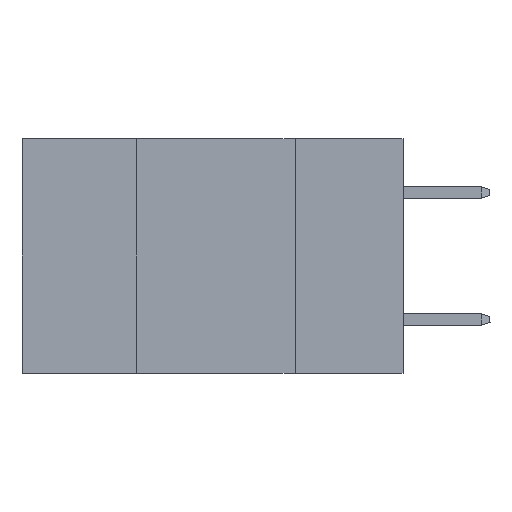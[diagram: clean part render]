
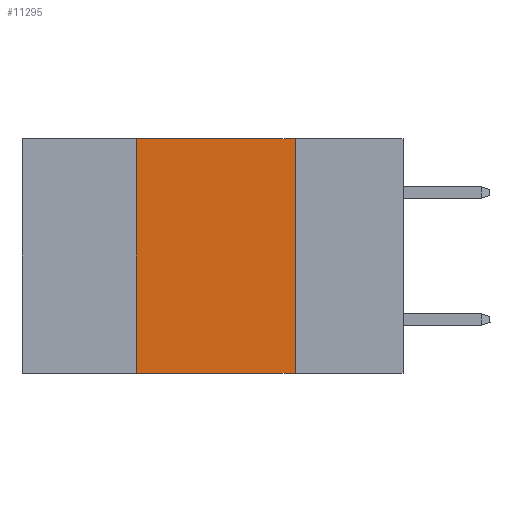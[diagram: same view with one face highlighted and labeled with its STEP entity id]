
A CAD part, left-side view. The second image highlights one B-rep face of the part: STEP entity #11295.
In plain terms, the highlighted planar face has unit normal (-1, 0, 0).
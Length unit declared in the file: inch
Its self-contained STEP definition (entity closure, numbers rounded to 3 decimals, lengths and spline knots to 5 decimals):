
#46 = CARTESIAN_POINT ( 'NONE',  ( 0., 0.42, -0.37 ) ) ;
#271 = ORIENTED_EDGE ( 'NONE', *, *, #1287, .F. ) ;
#534 = CARTESIAN_POINT ( 'NONE',  ( 0., 0.17, -0.37 ) ) ;
#814 = LINE ( 'NONE', #4712, #7866 ) ;
#1287 = EDGE_CURVE ( 'NONE', #6392, #10221, #2279, .T. ) ;
#1678 = CARTESIAN_POINT ( 'NONE',  ( 0., 0.6, 0. ) ) ;
#2162 = EDGE_LOOP ( 'NONE', ( #271, #5222, #3661, #5683 ) ) ;
#2279 = LINE ( 'NONE', #11916, #7397 ) ;
#2677 = LINE ( 'NONE', #10434, #7448 ) ;
#3661 = ORIENTED_EDGE ( 'NONE', *, *, #4582, .F. ) ;
#3765 = CARTESIAN_POINT ( 'NONE',  ( 0., 0.17, 0. ) ) ;
#4069 = VERTEX_POINT ( 'NONE', #46 ) ;
#4582 = EDGE_CURVE ( 'NONE', #4069, #7107, #12028, .T. ) ;
#4599 = DIRECTION ( 'NONE',  ( 0., 0., 1. ) ) ;
#4712 = CARTESIAN_POINT ( 'NONE',  ( 0., 0.6, 0. ) ) ;
#5222 = ORIENTED_EDGE ( 'NONE', *, *, #9831, .F. ) ;
#5490 = DIRECTION ( 'NONE',  ( 1., 0., 0. ) ) ;
#5683 = ORIENTED_EDGE ( 'NONE', *, *, #8972, .T. ) ;
#5736 = DIRECTION ( 'NONE',  ( 0., -1., 0. ) ) ;
#6145 = DIRECTION ( 'NONE',  ( 0., 0., -1. ) ) ;
#6288 = DIRECTION ( 'NONE',  ( 0., 0., -1. ) ) ;
#6392 = VERTEX_POINT ( 'NONE', #3765 ) ;
#7107 = VERTEX_POINT ( 'NONE', #11105 ) ;
#7129 = CARTESIAN_POINT ( 'NONE',  ( 0., 0.42, 0. ) ) ;
#7397 = VECTOR ( 'NONE', #6145, 39.37008 ) ;
#7409 = FACE_OUTER_BOUND ( 'NONE', #2162, .T. ) ;
#7448 = VECTOR ( 'NONE', #5736, 39.37008 ) ;
#7866 = VECTOR ( 'NONE', #8507, 39.37008 ) ;
#8507 = DIRECTION ( 'NONE',  ( 0., -1., 0. ) ) ;
#8911 = AXIS2_PLACEMENT_3D ( 'NONE', #1678, #5490, #6288 ) ;
#8972 = EDGE_CURVE ( 'NONE', #4069, #10221, #2677, .T. ) ;
#9831 = EDGE_CURVE ( 'NONE', #7107, #6392, #814, .T. ) ;
#10221 = VERTEX_POINT ( 'NONE', #534 ) ;
#10311 = PLANE ( 'NONE',  #8911 ) ;
#10434 = CARTESIAN_POINT ( 'NONE',  ( 0., 0.6, -0.37 ) ) ;
#10455 = VECTOR ( 'NONE', #4599, 39.37008 ) ;
#11105 = CARTESIAN_POINT ( 'NONE',  ( 0., 0.42, 0. ) ) ;
#11295 = ADVANCED_FACE ( 'NONE', ( #7409 ), #10311, .F. ) ;
#11916 = CARTESIAN_POINT ( 'NONE',  ( 0., 0.17, 0. ) ) ;
#12028 = LINE ( 'NONE', #7129, #10455 ) ;
